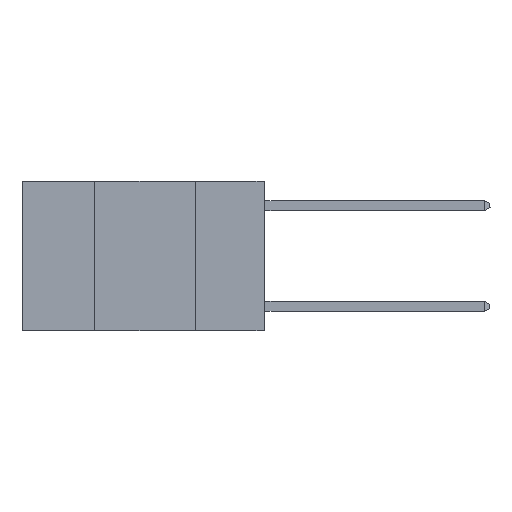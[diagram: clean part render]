
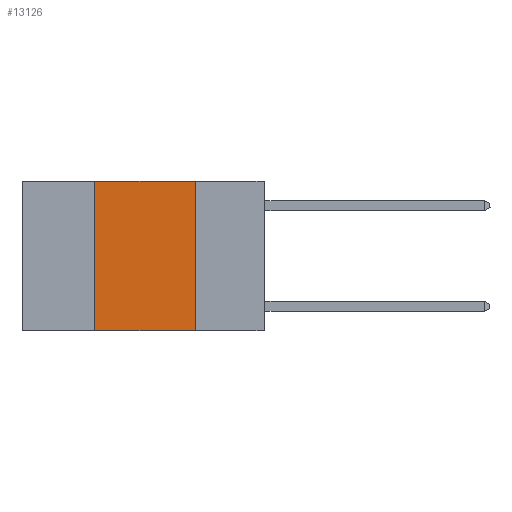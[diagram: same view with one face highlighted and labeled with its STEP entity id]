
A CAD part, left-side view. The second image highlights one B-rep face of the part: STEP entity #13126.
In plain terms, the highlighted planar face has unit normal (-1, 0, 0).
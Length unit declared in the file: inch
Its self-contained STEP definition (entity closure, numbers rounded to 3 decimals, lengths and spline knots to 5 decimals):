
#693 = DIRECTION ( 'NONE',  ( 0., 0., -1. ) ) ;
#1272 = ORIENTED_EDGE ( 'NONE', *, *, #15986, .F. ) ;
#1639 = ORIENTED_EDGE ( 'NONE', *, *, #8337, .F. ) ;
#2561 = LINE ( 'NONE', #9354, #5483 ) ;
#2760 = AXIS2_PLACEMENT_3D ( 'NONE', #15756, #8213, #693 ) ;
#3159 = DIRECTION ( 'NONE',  ( 0., 0., -1. ) ) ;
#4398 = CARTESIAN_POINT ( 'NONE',  ( 0., 0.42, 0. ) ) ;
#4592 = ORIENTED_EDGE ( 'NONE', *, *, #4744, .F. ) ;
#4744 = EDGE_CURVE ( 'NONE', #6045, #15906, #15564, .T. ) ;
#4992 = ORIENTED_EDGE ( 'NONE', *, *, #9845, .T. ) ;
#5203 = VECTOR ( 'NONE', #6027, 39.37008 ) ;
#5483 = VECTOR ( 'NONE', #3159, 39.37008 ) ;
#6027 = DIRECTION ( 'NONE',  ( 0., 0., 1. ) ) ;
#6045 = VERTEX_POINT ( 'NONE', #4398 ) ;
#6487 = VECTOR ( 'NONE', #7864, 39.37008 ) ;
#6894 = LINE ( 'NONE', #12956, #6487 ) ;
#6925 = FACE_OUTER_BOUND ( 'NONE', #13231, .T. ) ;
#7864 = DIRECTION ( 'NONE',  ( 0., -1., 0. ) ) ;
#8213 = DIRECTION ( 'NONE',  ( 1., 0., 0. ) ) ;
#8337 = EDGE_CURVE ( 'NONE', #16037, #6045, #8547, .T. ) ;
#8547 = LINE ( 'NONE', #14916, #5203 ) ;
#8622 = CARTESIAN_POINT ( 'NONE',  ( 0., 0.6, 0. ) ) ;
#8623 = CARTESIAN_POINT ( 'NONE',  ( 0., 0.17, -0.37 ) ) ;
#9230 = CARTESIAN_POINT ( 'NONE',  ( 0., 0.17, 0. ) ) ;
#9354 = CARTESIAN_POINT ( 'NONE',  ( 0., 0.17, 0. ) ) ;
#9845 = EDGE_CURVE ( 'NONE', #16037, #10231, #6894, .T. ) ;
#9901 = DIRECTION ( 'NONE',  ( 0., -1., 0. ) ) ;
#10231 = VERTEX_POINT ( 'NONE', #8623 ) ;
#11841 = VECTOR ( 'NONE', #9901, 39.37008 ) ;
#12037 = PLANE ( 'NONE',  #2760 ) ;
#12956 = CARTESIAN_POINT ( 'NONE',  ( 0., 0.6, -0.37 ) ) ;
#13126 = ADVANCED_FACE ( 'NONE', ( #6925 ), #12037, .F. ) ;
#13231 = EDGE_LOOP ( 'NONE', ( #1272, #4592, #1639, #4992 ) ) ;
#13354 = CARTESIAN_POINT ( 'NONE',  ( 0., 0.42, -0.37 ) ) ;
#14916 = CARTESIAN_POINT ( 'NONE',  ( 0., 0.42, 0. ) ) ;
#15564 = LINE ( 'NONE', #8622, #11841 ) ;
#15756 = CARTESIAN_POINT ( 'NONE',  ( 0., 0.6, 0. ) ) ;
#15906 = VERTEX_POINT ( 'NONE', #9230 ) ;
#15986 = EDGE_CURVE ( 'NONE', #15906, #10231, #2561, .T. ) ;
#16037 = VERTEX_POINT ( 'NONE', #13354 ) ;
